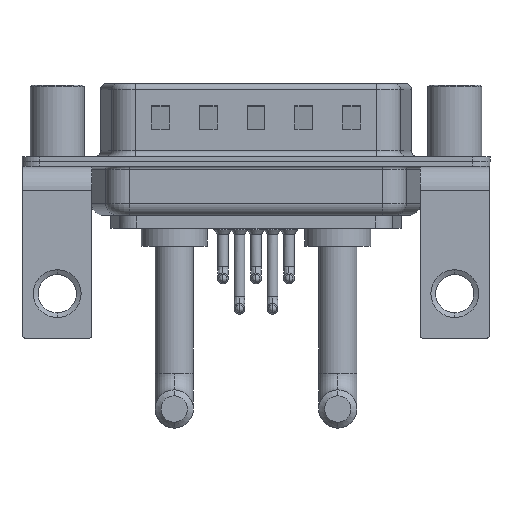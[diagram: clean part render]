
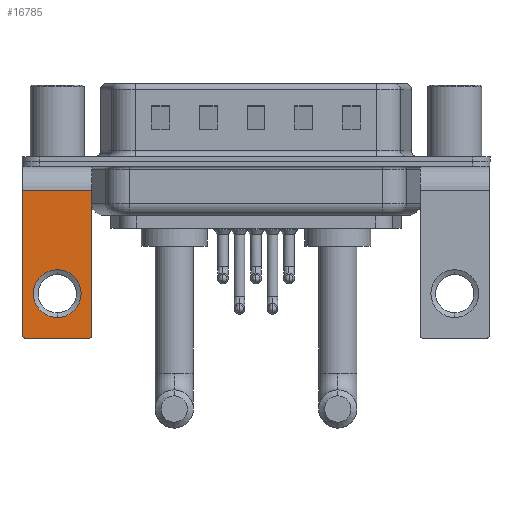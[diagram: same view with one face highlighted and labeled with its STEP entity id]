
A CAD part, front view. The second image highlights one B-rep face of the part: STEP entity #16785.
In plain terms, the highlighted planar face has unit normal (0, -1, 0).
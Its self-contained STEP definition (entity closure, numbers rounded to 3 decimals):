
#133 = CARTESIAN_POINT ( 'NONE',  ( 0., -6.25, -11.07 ) ) ;
#262 = DIRECTION ( 'NONE',  ( 0., 1., 0. ) ) ;
#523 = DIRECTION ( 'NONE',  ( 0., 0., -1. ) ) ;
#795 = AXIS2_PLACEMENT_3D ( 'NONE', #22639, #2835, #13748 ) ;
#868 = CARTESIAN_POINT ( 'NONE',  ( -2.9, -6.25, -2.4 ) ) ;
#916 = DIRECTION ( 'NONE',  ( 0., 1., 0. ) ) ;
#1262 = VERTEX_POINT ( 'NONE', #5855 ) ;
#1364 = CIRCLE ( 'NONE', #17637, 2. ) ;
#1475 = AXIS2_PLACEMENT_3D ( 'NONE', #15203, #15314, #22440 ) ;
#2050 = AXIS2_PLACEMENT_3D ( 'NONE', #133, #262, #7499 ) ;
#2051 = EDGE_CURVE ( 'NONE', #11189, #6044, #16049, .T. ) ;
#2063 = CIRCLE ( 'NONE', #17210, 0.25 ) ;
#2139 = DIRECTION ( 'NONE',  ( -1., 0., 0. ) ) ;
#2755 = LINE ( 'NONE', #868, #5634 ) ;
#2834 = CARTESIAN_POINT ( 'NONE',  ( 2.65, -6.25, -14.8 ) ) ;
#2835 = DIRECTION ( 'NONE',  ( 0., 1., 0. ) ) ;
#2925 = VERTEX_POINT ( 'NONE', #14203 ) ;
#2994 = CIRCLE ( 'NONE', #1475, 0.25 ) ;
#3144 = CARTESIAN_POINT ( 'NONE',  ( 2.9, -6.25, -14.55 ) ) ;
#3420 = ORIENTED_EDGE ( 'NONE', *, *, #9181, .T. ) ;
#3952 = VERTEX_POINT ( 'NONE', #2834 ) ;
#3957 = CARTESIAN_POINT ( 'NONE',  ( 2.9, -6.25, -2.4 ) ) ;
#4624 = LINE ( 'NONE', #15519, #9887 ) ;
#5052 = ORIENTED_EDGE ( 'NONE', *, *, #2051, .T. ) ;
#5502 = LINE ( 'NONE', #3957, #14197 ) ;
#5634 = VECTOR ( 'NONE', #16858, 1000. ) ;
#5822 = VECTOR ( 'NONE', #2139, 1000. ) ;
#5855 = CARTESIAN_POINT ( 'NONE',  ( 2.9, -6.25, -2.4 ) ) ;
#6044 = VERTEX_POINT ( 'NONE', #12033 ) ;
#6574 = VERTEX_POINT ( 'NONE', #22880 ) ;
#7355 = CARTESIAN_POINT ( 'NONE',  ( -2.65, -6.25, -14.55 ) ) ;
#7499 = DIRECTION ( 'NONE',  ( 0., 0., 1. ) ) ;
#8148 = DIRECTION ( 'NONE',  ( 0., 0., 1. ) ) ;
#8413 = DIRECTION ( 'NONE',  ( -1., 0., 0. ) ) ;
#8692 = ORIENTED_EDGE ( 'NONE', *, *, #21526, .T. ) ;
#9181 = EDGE_CURVE ( 'NONE', #6044, #11189, #1364, .T. ) ;
#9887 = VECTOR ( 'NONE', #8413, 1000. ) ;
#9964 = FACE_BOUND ( 'NONE', #18041, .T. ) ;
#10174 = CARTESIAN_POINT ( 'NONE',  ( 0., -6.25, -11.07 ) ) ;
#10198 = FACE_OUTER_BOUND ( 'NONE', #20787, .T. ) ;
#10374 = EDGE_CURVE ( 'NONE', #1262, #12762, #5502, .T. ) ;
#11189 = VERTEX_POINT ( 'NONE', #14534 ) ;
#12033 = CARTESIAN_POINT ( 'NONE',  ( 0., -6.25, -13.07 ) ) ;
#12762 = VERTEX_POINT ( 'NONE', #3144 ) ;
#12820 = ORIENTED_EDGE ( 'NONE', *, *, #10374, .F. ) ;
#13053 = DIRECTION ( 'NONE',  ( 0., 0., 1. ) ) ;
#13748 = DIRECTION ( 'NONE',  ( 0., 0., 1. ) ) ;
#14197 = VECTOR ( 'NONE', #523, 1000. ) ;
#14203 = CARTESIAN_POINT ( 'NONE',  ( -2.9, -6.25, -2.4 ) ) ;
#14534 = CARTESIAN_POINT ( 'NONE',  ( 0., -6.25, -9.07 ) ) ;
#14536 = ORIENTED_EDGE ( 'NONE', *, *, #20494, .F. ) ;
#15203 = CARTESIAN_POINT ( 'NONE',  ( 2.65, -6.25, -14.55 ) ) ;
#15314 = DIRECTION ( 'NONE',  ( 0., -1., 0. ) ) ;
#15519 = CARTESIAN_POINT ( 'NONE',  ( 2.9, -6.25, -2.4 ) ) ;
#15577 = ORIENTED_EDGE ( 'NONE', *, *, #17553, .T. ) ;
#16049 = CIRCLE ( 'NONE', #2050, 2. ) ;
#16785 = ADVANCED_FACE ( 'NONE', ( #9964, #10198 ), #17182, .F. ) ;
#16812 = EDGE_CURVE ( 'NONE', #1262, #2925, #4624, .T. ) ;
#16858 = DIRECTION ( 'NONE',  ( 0., 0., -1. ) ) ;
#17182 = PLANE ( 'NONE',  #795 ) ;
#17210 = AXIS2_PLACEMENT_3D ( 'NONE', #7355, #18264, #13053 ) ;
#17450 = EDGE_CURVE ( 'NONE', #2925, #6574, #2755, .T. ) ;
#17553 = EDGE_CURVE ( 'NONE', #3952, #12762, #2994, .T. ) ;
#17637 = AXIS2_PLACEMENT_3D ( 'NONE', #10174, #916, #8148 ) ;
#18041 = EDGE_LOOP ( 'NONE', ( #3420, #5052 ) ) ;
#18264 = DIRECTION ( 'NONE',  ( 0., -1., 0. ) ) ;
#18497 = LINE ( 'NONE', #22405, #5822 ) ;
#18617 = CARTESIAN_POINT ( 'NONE',  ( -2.65, -6.25, -14.8 ) ) ;
#20494 = EDGE_CURVE ( 'NONE', #3952, #21447, #18497, .T. ) ;
#20787 = EDGE_LOOP ( 'NONE', ( #23432, #8692, #14536, #15577, #12820, #22758 ) ) ;
#21447 = VERTEX_POINT ( 'NONE', #18617 ) ;
#21526 = EDGE_CURVE ( 'NONE', #6574, #21447, #2063, .T. ) ;
#22405 = CARTESIAN_POINT ( 'NONE',  ( 2.9, -6.25, -14.8 ) ) ;
#22440 = DIRECTION ( 'NONE',  ( 0., 0., 1. ) ) ;
#22639 = CARTESIAN_POINT ( 'NONE',  ( 2.9, -6.25, -2.4 ) ) ;
#22758 = ORIENTED_EDGE ( 'NONE', *, *, #16812, .T. ) ;
#22880 = CARTESIAN_POINT ( 'NONE',  ( -2.9, -6.25, -14.55 ) ) ;
#23432 = ORIENTED_EDGE ( 'NONE', *, *, #17450, .T. ) ;
